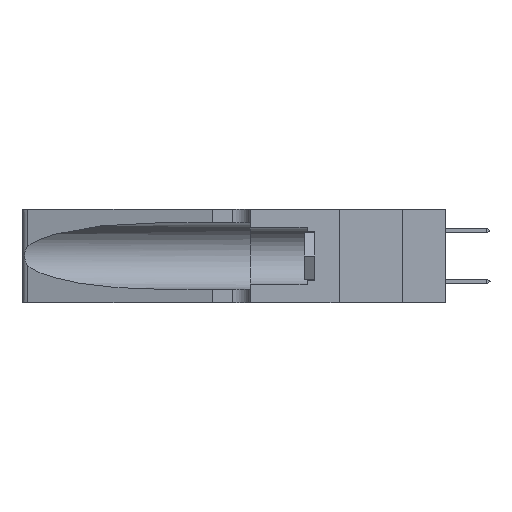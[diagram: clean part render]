
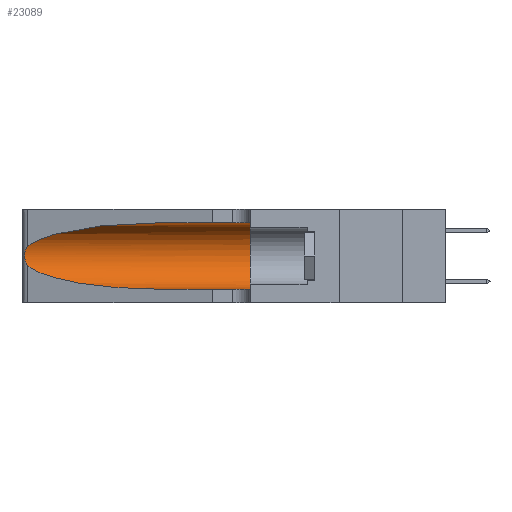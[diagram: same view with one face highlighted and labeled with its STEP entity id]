
A CAD part, left-side view. The second image highlights one B-rep face of the part: STEP entity #23089.
In plain terms, the highlighted cylindrical face has radius 3.308 mm (diameter 6.617 mm), a partial arc.
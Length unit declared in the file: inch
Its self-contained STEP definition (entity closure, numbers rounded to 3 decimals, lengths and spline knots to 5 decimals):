
#781 =( BOUNDED_CURVE ( )  B_SPLINE_CURVE ( 3, ( #11345, #6062, #31771, #16591 ),
 .UNSPECIFIED., .F., .F. ) 
 B_SPLINE_CURVE_WITH_KNOTS ( ( 4, 4 ),
 ( 1.5708, 2.84003 ),
 .UNSPECIFIED. ) 
 CURVE ( )  GEOMETRIC_REPRESENTATION_ITEM ( )  RATIONAL_B_SPLINE_CURVE ( ( 1., 0.87, 0.87, 1. ) ) 
 REPRESENTATION_ITEM ( '' )  );
#919 = CARTESIAN_POINT ( 'NONE',  ( 0.1305, 0.72297, 0.05475 ) ) ;
#1701 = VERTEX_POINT ( 'NONE', #11390 ) ;
#2606 = CARTESIAN_POINT ( 'NONE',  ( 0.26018, 1.23835, 0.19895 ) ) ;
#2969 = CIRCLE ( 'NONE', #29060, 0.13025 ) ;
#3643 = CARTESIAN_POINT ( 'NONE',  ( 0.25487, 1.22718, 0.22369 ) ) ;
#3843 = VERTEX_POINT ( 'NONE', #14903 ) ;
#4209 = DIRECTION ( 'NONE',  ( 0., 1., 0. ) ) ;
#4289 = DIRECTION ( 'NONE',  ( 0., -1., 0. ) ) ;
#4371 = B_SPLINE_CURVE_WITH_KNOTS ( 'NONE', 3,
 ( #23311, #28369, #15744, #19115, #18298, #2606, #20887, #5292, #23419, #7950, #25961, #10566, #28482, #13243 ),
 .UNSPECIFIED., .F., .F.,
 ( 4, 2, 2, 2, 2, 2, 4 ),
 ( 0., 0.00027, 0.00053, 0.00107, 0.0016, 0.00187, 0.00214 ),
 .UNSPECIFIED. ) ;
#5292 = CARTESIAN_POINT ( 'NONE',  ( 0.26075, 1.23896, 0.178 ) ) ;
#6062 = CARTESIAN_POINT ( 'NONE',  ( 0.18966, 0.96281, 0.31525 ) ) ;
#6385 = LINE ( 'NONE', #14453, #26162 ) ;
#6668 = VERTEX_POINT ( 'NONE', #29943 ) ;
#7950 = CARTESIAN_POINT ( 'NONE',  ( 0.25856, 1.23593, 0.16098 ) ) ;
#10566 = CARTESIAN_POINT ( 'NONE',  ( 0.25639, 1.23186, 0.15144 ) ) ;
#11345 = CARTESIAN_POINT ( 'NONE',  ( 0.1305, 0.72297, 0.31525 ) ) ;
#11390 = CARTESIAN_POINT ( 'NONE',  ( 0.1305, 0.72297, 0.05475 ) ) ;
#11793 = DIRECTION ( 'NONE',  ( 0., -1., 0. ) ) ;
#11967 = CARTESIAN_POINT ( 'NONE',  ( 0.1305, 1.61858, 0.31525 ) ) ;
#12031 = FACE_OUTER_BOUND ( 'NONE', #22606, .T. ) ;
#12141 = DIRECTION ( 'NONE',  ( 0., 0., -1. ) ) ;
#13243 = CARTESIAN_POINT ( 'NONE',  ( 0.25487, 1.22718, 0.14631 ) ) ;
#13718 = ORIENTED_EDGE ( 'NONE', *, *, #31955, .F. ) ;
#14453 = CARTESIAN_POINT ( 'NONE',  ( 0.1305, 1.61858, 0.05475 ) ) ;
#14628 = DIRECTION ( 'NONE',  ( 0., -1., 0. ) ) ;
#14891 = EDGE_CURVE ( 'NONE', #1701, #3843, #6385, .T. ) ;
#14903 = CARTESIAN_POINT ( 'NONE',  ( 0.1305, 0.35, 0.05475 ) ) ;
#15215 = VERTEX_POINT ( 'NONE', #15654 ) ;
#15654 = CARTESIAN_POINT ( 'NONE',  ( 0.1305, 0.35, 0.31525 ) ) ;
#15744 = CARTESIAN_POINT ( 'NONE',  ( 0.25639, 1.23184, 0.21858 ) ) ;
#16591 = CARTESIAN_POINT ( 'NONE',  ( 0.25487, 1.22718, 0.22369 ) ) ;
#16666 = CARTESIAN_POINT ( 'NONE',  ( 0.18966, 0.96281, 0.05475 ) ) ;
#17838 = VERTEX_POINT ( 'NONE', #3643 ) ;
#17957 = EDGE_CURVE ( 'NONE', #15215, #3843, #2969, .T. ) ;
#18298 = CARTESIAN_POINT ( 'NONE',  ( 0.25854, 1.2359, 0.20912 ) ) ;
#19115 = CARTESIAN_POINT ( 'NONE',  ( 0.25787, 1.23484, 0.2124 ) ) ;
#19861 = CARTESIAN_POINT ( 'NONE',  ( 0.1305, 0.35, 0.185 ) ) ;
#19945 = CARTESIAN_POINT ( 'NONE',  ( 0.1305, 1.61858, 0.185 ) ) ;
#20887 = CARTESIAN_POINT ( 'NONE',  ( 0.26075, 1.23896, 0.19203 ) ) ;
#20990 = EDGE_CURVE ( 'NONE', #6668, #17838, #781, .T. ) ;
#21022 = CARTESIAN_POINT ( 'NONE',  ( 0.25487, 1.22718, 0.14631 ) ) ;
#22397 = DIRECTION ( 'NONE',  ( 0., 0., 1. ) ) ;
#22502 =( BOUNDED_CURVE ( )  B_SPLINE_CURVE ( 3, ( #29313, #31854, #16666, #919 ),
 .UNSPECIFIED., .F., .F. ) 
 B_SPLINE_CURVE_WITH_KNOTS ( ( 4, 4 ),
 ( 3.44316, 4.71239 ),
 .UNSPECIFIED. ) 
 CURVE ( )  GEOMETRIC_REPRESENTATION_ITEM ( )  RATIONAL_B_SPLINE_CURVE ( ( 1., 0.87, 0.87, 1. ) ) 
 REPRESENTATION_ITEM ( '' )  );
#22606 = EDGE_LOOP ( 'NONE', ( #30625, #23683, #29035, #29246, #32220, #13718 ) ) ;
#23089 = ADVANCED_FACE ( 'NONE', ( #12031 ), #24863, .F. ) ;
#23311 = CARTESIAN_POINT ( 'NONE',  ( 0.25487, 1.22718, 0.22369 ) ) ;
#23419 = CARTESIAN_POINT ( 'NONE',  ( 0.26017, 1.23833, 0.17102 ) ) ;
#23683 = ORIENTED_EDGE ( 'NONE', *, *, #28449, .T. ) ;
#24505 = VECTOR ( 'NONE', #14628, 39.37008 ) ;
#24664 = EDGE_CURVE ( 'NONE', #31613, #1701, #22502, .T. ) ;
#24863 = CYLINDRICAL_SURFACE ( 'NONE', #31297, 0.13025 ) ;
#25961 = CARTESIAN_POINT ( 'NONE',  ( 0.25789, 1.23486, 0.15765 ) ) ;
#26162 = VECTOR ( 'NONE', #11793, 39.37008 ) ;
#28369 = CARTESIAN_POINT ( 'NONE',  ( 0.25555, 1.22994, 0.2215 ) ) ;
#28449 = EDGE_CURVE ( 'NONE', #17838, #31613, #4371, .T. ) ;
#28482 = CARTESIAN_POINT ( 'NONE',  ( 0.25555, 1.22993, 0.14849 ) ) ;
#29035 = ORIENTED_EDGE ( 'NONE', *, *, #24664, .T. ) ;
#29060 = AXIS2_PLACEMENT_3D ( 'NONE', #19861, #4209, #22397 ) ;
#29246 = ORIENTED_EDGE ( 'NONE', *, *, #14891, .T. ) ;
#29313 = CARTESIAN_POINT ( 'NONE',  ( 0.25487, 1.22718, 0.14631 ) ) ;
#29943 = CARTESIAN_POINT ( 'NONE',  ( 0.1305, 0.72297, 0.31525 ) ) ;
#30625 = ORIENTED_EDGE ( 'NONE', *, *, #20990, .T. ) ;
#31297 = AXIS2_PLACEMENT_3D ( 'NONE', #19945, #4289, #12141 ) ;
#31613 = VERTEX_POINT ( 'NONE', #21022 ) ;
#31771 = CARTESIAN_POINT ( 'NONE',  ( 0.2373, 1.15595, 0.28018 ) ) ;
#31854 = CARTESIAN_POINT ( 'NONE',  ( 0.2373, 1.15595, 0.08982 ) ) ;
#31955 = EDGE_CURVE ( 'NONE', #6668, #15215, #32012, .T. ) ;
#32012 = LINE ( 'NONE', #11967, #24505 ) ;
#32220 = ORIENTED_EDGE ( 'NONE', *, *, #17957, .F. ) ;
